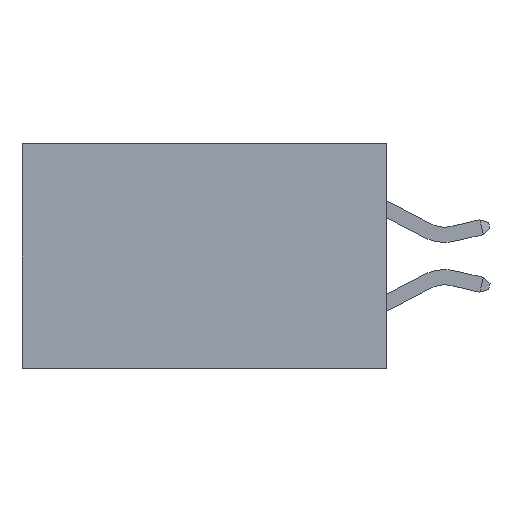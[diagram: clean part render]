
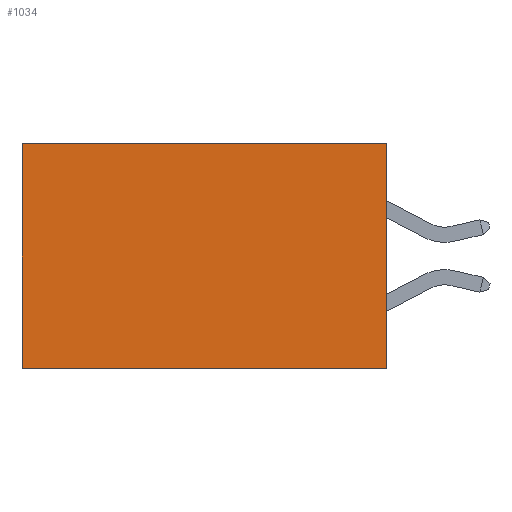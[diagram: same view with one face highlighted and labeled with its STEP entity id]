
A CAD part, left-side view. The second image highlights one B-rep face of the part: STEP entity #1034.
In plain terms, the highlighted planar face has unit normal (-1, 0, 0).
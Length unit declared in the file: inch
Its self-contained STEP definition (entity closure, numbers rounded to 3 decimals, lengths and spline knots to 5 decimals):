
#32 = VERTEX_POINT ( 'NONE', #5083 ) ;
#428 = AXIS2_PLACEMENT_3D ( 'NONE', #5092, #5035, #4962 ) ;
#1034 = ADVANCED_FACE ( 'NONE', ( #11347 ), #5453, .F. ) ;
#1317 = EDGE_CURVE ( 'NONE', #32, #15570, #6351, .T. ) ;
#2203 = EDGE_CURVE ( 'NONE', #10719, #3546, #17874, .T. ) ;
#2513 = VECTOR ( 'NONE', #16922, 39.37008 ) ;
#3157 = ORIENTED_EDGE ( 'NONE', *, *, #1317, .F. ) ;
#3546 = VERTEX_POINT ( 'NONE', #8108 ) ;
#4760 = EDGE_CURVE ( 'NONE', #3546, #15570, #13509, .T. ) ;
#4962 = DIRECTION ( 'NONE',  ( 0., 0., -1. ) ) ;
#5035 = DIRECTION ( 'NONE',  ( 1., 0., 0. ) ) ;
#5083 = CARTESIAN_POINT ( 'NONE',  ( 0.2615, 0., -0.37 ) ) ;
#5092 = CARTESIAN_POINT ( 'NONE',  ( 0.2615, 0., -0.37 ) ) ;
#5453 = PLANE ( 'NONE',  #428 ) ;
#6351 = LINE ( 'NONE', #17900, #2513 ) ;
#7825 = ORIENTED_EDGE ( 'NONE', *, *, #16191, .F. ) ;
#8108 = CARTESIAN_POINT ( 'NONE',  ( 0.2615, 0.6, 0. ) ) ;
#8718 = CARTESIAN_POINT ( 'NONE',  ( 0.2615, 0., -0.37 ) ) ;
#10102 = DIRECTION ( 'NONE',  ( 0., 0., -1. ) ) ;
#10152 = VECTOR ( 'NONE', #14040, 39.37008 ) ;
#10353 = CARTESIAN_POINT ( 'NONE',  ( 0.2615, 0.6, -0.37 ) ) ;
#10719 = VERTEX_POINT ( 'NONE', #12981 ) ;
#11347 = FACE_OUTER_BOUND ( 'NONE', #13105, .T. ) ;
#11738 = VECTOR ( 'NONE', #15963, 39.37008 ) ;
#12981 = CARTESIAN_POINT ( 'NONE',  ( 0.2615, 0., 0. ) ) ;
#13105 = EDGE_LOOP ( 'NONE', ( #15607, #3157, #7825, #16320 ) ) ;
#13509 = LINE ( 'NONE', #10353, #13971 ) ;
#13971 = VECTOR ( 'NONE', #10102, 39.37008 ) ;
#14040 = DIRECTION ( 'NONE',  ( 0., 1., 0. ) ) ;
#14360 = CARTESIAN_POINT ( 'NONE',  ( 0.2615, 0., 0. ) ) ;
#15570 = VERTEX_POINT ( 'NONE', #16164 ) ;
#15607 = ORIENTED_EDGE ( 'NONE', *, *, #4760, .T. ) ;
#15963 = DIRECTION ( 'NONE',  ( 0., 0., -1. ) ) ;
#16055 = LINE ( 'NONE', #8718, #11738 ) ;
#16164 = CARTESIAN_POINT ( 'NONE',  ( 0.2615, 0.6, -0.37 ) ) ;
#16191 = EDGE_CURVE ( 'NONE', #10719, #32, #16055, .T. ) ;
#16320 = ORIENTED_EDGE ( 'NONE', *, *, #2203, .T. ) ;
#16922 = DIRECTION ( 'NONE',  ( 0., 1., 0. ) ) ;
#17874 = LINE ( 'NONE', #14360, #10152 ) ;
#17900 = CARTESIAN_POINT ( 'NONE',  ( 0.2615, 0., -0.37 ) ) ;
